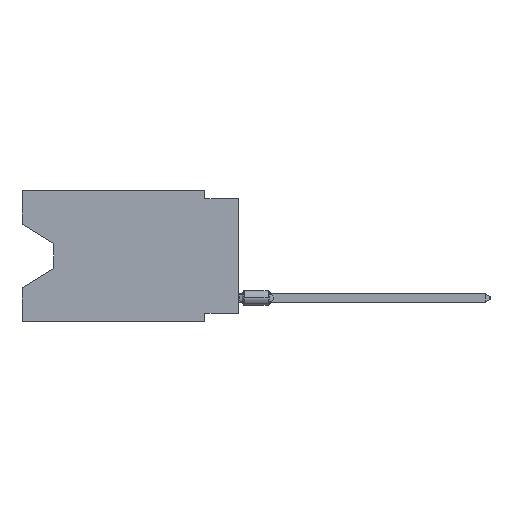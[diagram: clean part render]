
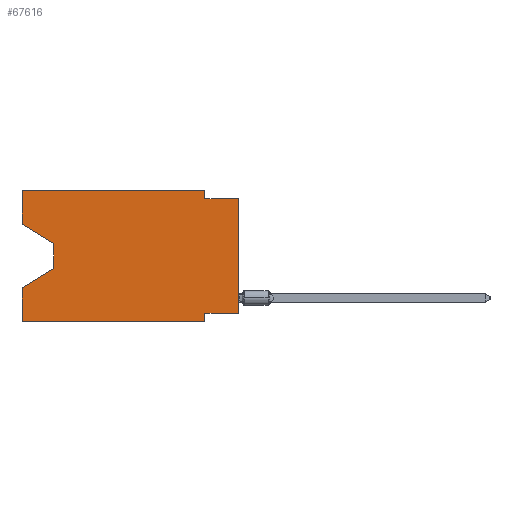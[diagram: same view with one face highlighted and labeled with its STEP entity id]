
A CAD part, left-side view. The second image highlights one B-rep face of the part: STEP entity #67616.
In plain terms, the highlighted planar face has unit normal (-1, 0, 0).
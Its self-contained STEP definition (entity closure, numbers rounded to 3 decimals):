
#39 = DIRECTION ( 'NONE',  ( 0., -0.855, -0.519 ) ) ;
#55 = LINE ( 'NONE', #28099, #67349 ) ;
#75 = ORIENTED_EDGE ( 'NONE', *, *, #35203, .F. ) ;
#223 = EDGE_CURVE ( 'NONE', #2593, #740, #10585, .T. ) ;
#740 = VERTEX_POINT ( 'NONE', #2576 ) ;
#1690 = EDGE_CURVE ( 'NONE', #59856, #55548, #54776, .T. ) ;
#2519 = CARTESIAN_POINT ( 'NONE',  ( 0., 2.54, 0. ) ) ;
#2576 = CARTESIAN_POINT ( 'NONE',  ( 0., 16.383, -7.36 ) ) ;
#2593 = VERTEX_POINT ( 'NONE', #16865 ) ;
#4830 = LINE ( 'NONE', #42179, #23603 ) ;
#6265 = DIRECTION ( 'NONE',  ( 0., 0., -1. ) ) ;
#6541 = EDGE_CURVE ( 'NONE', #41038, #20955, #67009, .T. ) ;
#7271 = ORIENTED_EDGE ( 'NONE', *, *, #23750, .F. ) ;
#7822 = EDGE_CURVE ( 'NONE', #70063, #38795, #51725, .T. ) ;
#8742 = EDGE_CURVE ( 'NONE', #10233, #51861, #35216, .T. ) ;
#9124 = ORIENTED_EDGE ( 'NONE', *, *, #63518, .F. ) ;
#10021 = ORIENTED_EDGE ( 'NONE', *, *, #8742, .T. ) ;
#10233 = VERTEX_POINT ( 'NONE', #53583 ) ;
#10585 = LINE ( 'NONE', #38331, #54977 ) ;
#11276 = ORIENTED_EDGE ( 'NONE', *, *, #17762, .F. ) ;
#11726 = DIRECTION ( 'NONE',  ( 0., 0., -1. ) ) ;
#11789 = CARTESIAN_POINT ( 'NONE',  ( 0., 0., 0. ) ) ;
#11963 = VECTOR ( 'NONE', #31934, 1000. ) ;
#14001 = DIRECTION ( 'NONE',  ( 0., -1., 0. ) ) ;
#15140 = PLANE ( 'NONE',  #59069 ) ;
#16425 = ORIENTED_EDGE ( 'NONE', *, *, #223, .T. ) ;
#16795 = VECTOR ( 'NONE', #55556, 1000. ) ;
#16865 = CARTESIAN_POINT ( 'NONE',  ( 0., 13.97, -5.893 ) ) ;
#17762 = EDGE_CURVE ( 'NONE', #20955, #51861, #55, .T. ) ;
#17913 = CARTESIAN_POINT ( 'NONE',  ( 0., 0., -9.271 ) ) ;
#19954 = CARTESIAN_POINT ( 'NONE',  ( 0., 2.54, -0.635 ) ) ;
#20688 = EDGE_LOOP ( 'NONE', ( #43754, #36990, #16425, #75, #10021, #11276, #25768, #39880, #44030, #9124, #50106, #7271 ) ) ;
#20955 = VERTEX_POINT ( 'NONE', #35291 ) ;
#21121 = VERTEX_POINT ( 'NONE', #19954 ) ;
#21606 = DIRECTION ( 'NONE',  ( 0., 0.855, -0.519 ) ) ;
#22784 = VECTOR ( 'NONE', #39852, 1000. ) ;
#23603 = VECTOR ( 'NONE', #36834, 1000. ) ;
#23750 = EDGE_CURVE ( 'NONE', #59856, #70063, #4830, .T. ) ;
#23845 = CARTESIAN_POINT ( 'NONE',  ( 0., 13.97, -4.013 ) ) ;
#24170 = CARTESIAN_POINT ( 'NONE',  ( 0., 16.383, -2.546 ) ) ;
#24597 = EDGE_CURVE ( 'NONE', #21121, #26418, #31334, .T. ) ;
#25768 = ORIENTED_EDGE ( 'NONE', *, *, #6541, .F. ) ;
#26418 = VERTEX_POINT ( 'NONE', #57567 ) ;
#27261 = CARTESIAN_POINT ( 'NONE',  ( 0., 13.97, -4.013 ) ) ;
#28099 = CARTESIAN_POINT ( 'NONE',  ( 0., 2.54, -9.906 ) ) ;
#31334 = LINE ( 'NONE', #62993, #65504 ) ;
#31934 = DIRECTION ( 'NONE',  ( 0., 0., 1. ) ) ;
#32378 = VECTOR ( 'NONE', #39, 1000. ) ;
#33199 = CARTESIAN_POINT ( 'NONE',  ( 0., 16.383, 0. ) ) ;
#34065 = VECTOR ( 'NONE', #14001, 1000. ) ;
#34194 = CARTESIAN_POINT ( 'NONE',  ( 0., 2.54, -9.906 ) ) ;
#35203 = EDGE_CURVE ( 'NONE', #10233, #740, #42594, .T. ) ;
#35216 = LINE ( 'NONE', #66891, #22784 ) ;
#35291 = CARTESIAN_POINT ( 'NONE',  ( 0., 2.54, -9.271 ) ) ;
#36834 = DIRECTION ( 'NONE',  ( 0., 0., 1. ) ) ;
#36990 = ORIENTED_EDGE ( 'NONE', *, *, #68838, .T. ) ;
#38331 = CARTESIAN_POINT ( 'NONE',  ( 0., 13.97, -5.893 ) ) ;
#38795 = VERTEX_POINT ( 'NONE', #64910 ) ;
#39852 = DIRECTION ( 'NONE',  ( 0., -1., 0. ) ) ;
#39880 = ORIENTED_EDGE ( 'NONE', *, *, #42166, .T. ) ;
#41038 = VERTEX_POINT ( 'NONE', #52569 ) ;
#42166 = EDGE_CURVE ( 'NONE', #41038, #26418, #60539, .T. ) ;
#42168 = VECTOR ( 'NONE', #6265, 1000. ) ;
#42179 = CARTESIAN_POINT ( 'NONE',  ( 0., 16.383, 0. ) ) ;
#42594 = LINE ( 'NONE', #69635, #11963 ) ;
#43091 = VECTOR ( 'NONE', #55280, 1000. ) ;
#43754 = ORIENTED_EDGE ( 'NONE', *, *, #1690, .T. ) ;
#44030 = ORIENTED_EDGE ( 'NONE', *, *, #24597, .F. ) ;
#45184 = LINE ( 'NONE', #2519, #49692 ) ;
#45334 = CARTESIAN_POINT ( 'NONE',  ( 0., 16.383, 0. ) ) ;
#45531 = DIRECTION ( 'NONE',  ( 0., 0., -1. ) ) ;
#49553 = DIRECTION ( 'NONE',  ( 1., 0., 0. ) ) ;
#49692 = VECTOR ( 'NONE', #45531, 1000. ) ;
#50106 = ORIENTED_EDGE ( 'NONE', *, *, #7822, .F. ) ;
#50685 = CARTESIAN_POINT ( 'NONE',  ( 0., 16.383, 0. ) ) ;
#51725 = LINE ( 'NONE', #50685, #34065 ) ;
#51861 = VERTEX_POINT ( 'NONE', #34194 ) ;
#52569 = CARTESIAN_POINT ( 'NONE',  ( 0., 0., -9.271 ) ) ;
#53583 = CARTESIAN_POINT ( 'NONE',  ( 0., 16.383, -9.906 ) ) ;
#54776 = LINE ( 'NONE', #65096, #32378 ) ;
#54977 = VECTOR ( 'NONE', #21606, 1000. ) ;
#54998 = LINE ( 'NONE', #27261, #42168 ) ;
#55280 = DIRECTION ( 'NONE',  ( 0., 1., 0. ) ) ;
#55548 = VERTEX_POINT ( 'NONE', #23845 ) ;
#55556 = DIRECTION ( 'NONE',  ( 0., 0., 1. ) ) ;
#57567 = CARTESIAN_POINT ( 'NONE',  ( 0., 0., -0.635 ) ) ;
#57652 = DIRECTION ( 'NONE',  ( 0., -1., 0. ) ) ;
#59069 = AXIS2_PLACEMENT_3D ( 'NONE', #33199, #49553, #65923 ) ;
#59856 = VERTEX_POINT ( 'NONE', #24170 ) ;
#60539 = LINE ( 'NONE', #11789, #16795 ) ;
#60578 = FACE_OUTER_BOUND ( 'NONE', #20688, .T. ) ;
#62993 = CARTESIAN_POINT ( 'NONE',  ( 0., 0., -0.635 ) ) ;
#63518 = EDGE_CURVE ( 'NONE', #38795, #21121, #45184, .T. ) ;
#64910 = CARTESIAN_POINT ( 'NONE',  ( 0., 2.54, 0. ) ) ;
#65096 = CARTESIAN_POINT ( 'NONE',  ( 0., 16.383, -2.546 ) ) ;
#65504 = VECTOR ( 'NONE', #57652, 1000. ) ;
#65923 = DIRECTION ( 'NONE',  ( 0., 0., -1. ) ) ;
#66891 = CARTESIAN_POINT ( 'NONE',  ( 0., 16.383, -9.906 ) ) ;
#67009 = LINE ( 'NONE', #17913, #43091 ) ;
#67349 = VECTOR ( 'NONE', #11726, 1000. ) ;
#67616 = ADVANCED_FACE ( 'NONE', ( #60578 ), #15140, .F. ) ;
#68838 = EDGE_CURVE ( 'NONE', #55548, #2593, #54998, .T. ) ;
#69635 = CARTESIAN_POINT ( 'NONE',  ( 0., 16.383, 0. ) ) ;
#70063 = VERTEX_POINT ( 'NONE', #45334 ) ;
